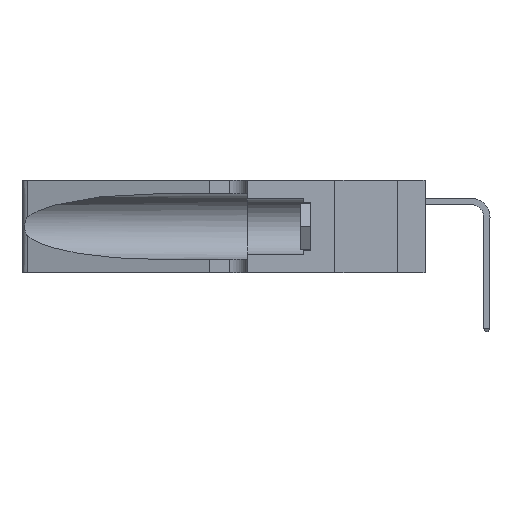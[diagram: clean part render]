
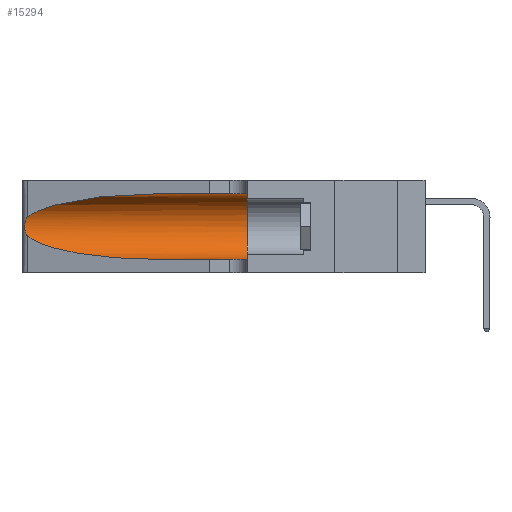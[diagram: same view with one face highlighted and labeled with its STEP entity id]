
A CAD part, left-side view. The second image highlights one B-rep face of the part: STEP entity #15294.
In plain terms, the highlighted cylindrical face has radius 3.308 mm (diameter 6.617 mm), a partial arc.
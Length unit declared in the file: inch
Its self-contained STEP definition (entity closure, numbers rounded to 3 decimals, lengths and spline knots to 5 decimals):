
#779 = EDGE_CURVE ( 'NONE', #27573, #32882, #19002, .T. ) ;
#1271 = CIRCLE ( 'NONE', #12718, 0.13025 ) ;
#1634 = ORIENTED_EDGE ( 'NONE', *, *, #13178, .T. ) ;
#1802 = CARTESIAN_POINT ( 'NONE',  ( 0.1305, 0.35, 0.185 ) ) ;
#2498 = CARTESIAN_POINT ( 'NONE',  ( 0.1305, 0.35, 0.05475 ) ) ;
#2604 = CARTESIAN_POINT ( 'NONE',  ( 0.1305, 0.72297, 0.05475 ) ) ;
#3843 = CARTESIAN_POINT ( 'NONE',  ( 0.1305, 0.35, 0.31525 ) ) ;
#4211 = ORIENTED_EDGE ( 'NONE', *, *, #779, .T. ) ;
#4695 = CARTESIAN_POINT ( 'NONE',  ( 0.25787, 1.23484, 0.2124 ) ) ;
#4702 = DIRECTION ( 'NONE',  ( 0., 0., 1. ) ) ;
#6024 = EDGE_LOOP ( 'NONE', ( #4211, #26231, #1634, #16131, #14676, #22324 ) ) ;
#6124 = DIRECTION ( 'NONE',  ( 0., -1., 0. ) ) ;
#6864 = DIRECTION ( 'NONE',  ( 0., -1., 0. ) ) ;
#7049 = CARTESIAN_POINT ( 'NONE',  ( 0.1305, 1.61858, 0.05475 ) ) ;
#7597 = CARTESIAN_POINT ( 'NONE',  ( 0.26018, 1.23835, 0.19895 ) ) ;
#9110 = CARTESIAN_POINT ( 'NONE',  ( 0.2373, 1.15595, 0.28018 ) ) ;
#9966 = DIRECTION ( 'NONE',  ( 0., -1., 0. ) ) ;
#10516 = CARTESIAN_POINT ( 'NONE',  ( 0.26075, 1.23896, 0.178 ) ) ;
#11048 = EDGE_CURVE ( 'NONE', #32055, #22278, #16496, .T. ) ;
#11796 = CARTESIAN_POINT ( 'NONE',  ( 0.1305, 0.72297, 0.31525 ) ) ;
#12718 = AXIS2_PLACEMENT_3D ( 'NONE', #1802, #21996, #4702 ) ;
#13178 = EDGE_CURVE ( 'NONE', #21157, #32055, #31326, .T. ) ;
#13431 = CARTESIAN_POINT ( 'NONE',  ( 0.25856, 1.23593, 0.16098 ) ) ;
#13515 = EDGE_CURVE ( 'NONE', #27573, #18231, #15839, .T. ) ;
#14113 = CARTESIAN_POINT ( 'NONE',  ( 0.18966, 0.96281, 0.05475 ) ) ;
#14676 = ORIENTED_EDGE ( 'NONE', *, *, #20583, .F. ) ;
#15294 = ADVANCED_FACE ( 'NONE', ( #27342 ), #33045, .F. ) ;
#15839 = LINE ( 'NONE', #21280, #22587 ) ;
#16131 = ORIENTED_EDGE ( 'NONE', *, *, #11048, .T. ) ;
#16202 = CARTESIAN_POINT ( 'NONE',  ( 0.25555, 1.22994, 0.2215 ) ) ;
#16327 = CARTESIAN_POINT ( 'NONE',  ( 0.25639, 1.23186, 0.15144 ) ) ;
#16496 = LINE ( 'NONE', #7049, #30763 ) ;
#17163 = B_SPLINE_CURVE_WITH_KNOTS ( 'NONE', 3,
 ( #36077, #16202, #21984, #4695, #24862, #7597, #27724, #10516, #30556, #13431, #33363, #16327, #36195, #19244 ),
 .UNSPECIFIED., .F., .F.,
 ( 4, 2, 2, 2, 2, 2, 4 ),
 ( 0., 0.00027, 0.00053, 0.00107, 0.0016, 0.00187, 0.00214 ),
 .UNSPECIFIED. ) ;
#17833 = CARTESIAN_POINT ( 'NONE',  ( 0.25487, 1.22718, 0.22369 ) ) ;
#18231 = VERTEX_POINT ( 'NONE', #3843 ) ;
#18424 = AXIS2_PLACEMENT_3D ( 'NONE', #23379, #6124, #26271 ) ;
#19002 =( BOUNDED_CURVE ( )  B_SPLINE_CURVE ( 3, ( #34827, #29180, #9110, #17833 ),
 .UNSPECIFIED., .F., .F. ) 
 B_SPLINE_CURVE_WITH_KNOTS ( ( 4, 4 ),
 ( 1.5708, 2.84003 ),
 .UNSPECIFIED. ) 
 CURVE ( )  GEOMETRIC_REPRESENTATION_ITEM ( )  RATIONAL_B_SPLINE_CURVE ( ( 1., 0.87, 0.87, 1. ) ) 
 REPRESENTATION_ITEM ( '' )  );
#19244 = CARTESIAN_POINT ( 'NONE',  ( 0.25487, 1.22718, 0.14631 ) ) ;
#19805 = CARTESIAN_POINT ( 'NONE',  ( 0.2373, 1.15595, 0.08982 ) ) ;
#19925 = CARTESIAN_POINT ( 'NONE',  ( 0.25487, 1.22718, 0.14631 ) ) ;
#20583 = EDGE_CURVE ( 'NONE', #18231, #22278, #1271, .T. ) ;
#21157 = VERTEX_POINT ( 'NONE', #24451 ) ;
#21280 = CARTESIAN_POINT ( 'NONE',  ( 0.1305, 1.61858, 0.31525 ) ) ;
#21984 = CARTESIAN_POINT ( 'NONE',  ( 0.25639, 1.23184, 0.21858 ) ) ;
#21996 = DIRECTION ( 'NONE',  ( 0., 1., 0. ) ) ;
#22278 = VERTEX_POINT ( 'NONE', #2498 ) ;
#22324 = ORIENTED_EDGE ( 'NONE', *, *, #13515, .F. ) ;
#22587 = VECTOR ( 'NONE', #6864, 39.37008 ) ;
#23379 = CARTESIAN_POINT ( 'NONE',  ( 0.1305, 1.61858, 0.185 ) ) ;
#24451 = CARTESIAN_POINT ( 'NONE',  ( 0.25487, 1.22718, 0.14631 ) ) ;
#24579 = CARTESIAN_POINT ( 'NONE',  ( 0.25487, 1.22718, 0.22369 ) ) ;
#24862 = CARTESIAN_POINT ( 'NONE',  ( 0.25854, 1.2359, 0.20912 ) ) ;
#26231 = ORIENTED_EDGE ( 'NONE', *, *, #35432, .T. ) ;
#26271 = DIRECTION ( 'NONE',  ( 0., 0., -1. ) ) ;
#27342 = FACE_OUTER_BOUND ( 'NONE', #6024, .T. ) ;
#27573 = VERTEX_POINT ( 'NONE', #11796 ) ;
#27724 = CARTESIAN_POINT ( 'NONE',  ( 0.26075, 1.23896, 0.19203 ) ) ;
#29180 = CARTESIAN_POINT ( 'NONE',  ( 0.18966, 0.96281, 0.31525 ) ) ;
#29480 = CARTESIAN_POINT ( 'NONE',  ( 0.1305, 0.72297, 0.05475 ) ) ;
#30556 = CARTESIAN_POINT ( 'NONE',  ( 0.26017, 1.23833, 0.17102 ) ) ;
#30763 = VECTOR ( 'NONE', #9966, 39.37008 ) ;
#31326 =( BOUNDED_CURVE ( )  B_SPLINE_CURVE ( 3, ( #19925, #19805, #14113, #2604 ),
 .UNSPECIFIED., .F., .F. ) 
 B_SPLINE_CURVE_WITH_KNOTS ( ( 4, 4 ),
 ( 3.44316, 4.71239 ),
 .UNSPECIFIED. ) 
 CURVE ( )  GEOMETRIC_REPRESENTATION_ITEM ( )  RATIONAL_B_SPLINE_CURVE ( ( 1., 0.87, 0.87, 1. ) ) 
 REPRESENTATION_ITEM ( '' )  );
#32055 = VERTEX_POINT ( 'NONE', #29480 ) ;
#32882 = VERTEX_POINT ( 'NONE', #24579 ) ;
#33045 = CYLINDRICAL_SURFACE ( 'NONE', #18424, 0.13025 ) ;
#33363 = CARTESIAN_POINT ( 'NONE',  ( 0.25789, 1.23486, 0.15765 ) ) ;
#34827 = CARTESIAN_POINT ( 'NONE',  ( 0.1305, 0.72297, 0.31525 ) ) ;
#35432 = EDGE_CURVE ( 'NONE', #32882, #21157, #17163, .T. ) ;
#36077 = CARTESIAN_POINT ( 'NONE',  ( 0.25487, 1.22718, 0.22369 ) ) ;
#36195 = CARTESIAN_POINT ( 'NONE',  ( 0.25555, 1.22993, 0.14849 ) ) ;
